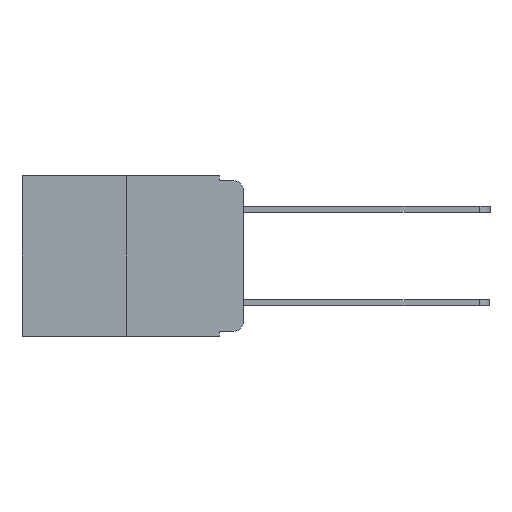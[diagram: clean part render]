
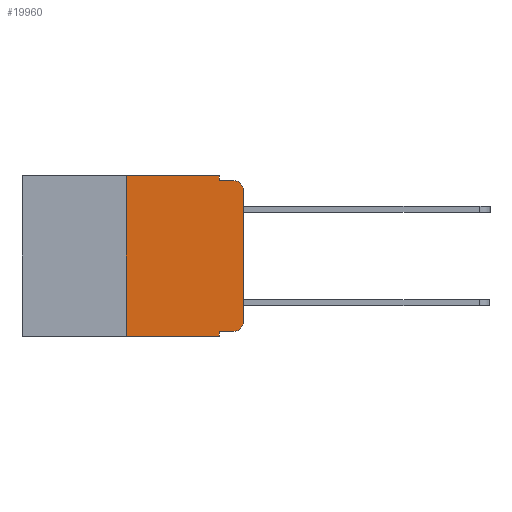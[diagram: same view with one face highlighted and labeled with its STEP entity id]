
A CAD part, left-side view. The second image highlights one B-rep face of the part: STEP entity #19960.
In plain terms, the highlighted planar face has unit normal (-1, 0, 0).
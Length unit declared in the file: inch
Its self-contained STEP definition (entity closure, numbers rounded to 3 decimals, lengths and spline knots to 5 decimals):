
#76 = LINE ( 'NONE', #2492, #4510 ) ;
#156 = ORIENTED_EDGE ( 'NONE', *, *, #2588, .F. ) ;
#288 = CARTESIAN_POINT ( 'NONE',  ( 0., 0.051, 0. ) ) ;
#314 = EDGE_CURVE ( 'NONE', #11053, #2908, #867, .T. ) ;
#435 = DIRECTION ( 'NONE',  ( 0., 0., -1. ) ) ;
#867 = CIRCLE ( 'NONE', #7590, 0.02 ) ;
#887 = CARTESIAN_POINT ( 'NONE',  ( 0., 0., 0. ) ) ;
#1005 = VERTEX_POINT ( 'NONE', #15264 ) ;
#1090 = CARTESIAN_POINT ( 'NONE',  ( 0., 0.051, -0.333 ) ) ;
#1467 = EDGE_CURVE ( 'NONE', #4015, #11053, #2107, .T. ) ;
#2075 = ORIENTED_EDGE ( 'NONE', *, *, #9707, .T. ) ;
#2107 = LINE ( 'NONE', #20034, #14259 ) ;
#2492 = CARTESIAN_POINT ( 'NONE',  ( 0., 0.051, -0.01 ) ) ;
#2574 = DIRECTION ( 'NONE',  ( 0., 0., 1. ) ) ;
#2588 = EDGE_CURVE ( 'NONE', #4015, #8609, #17088, .T. ) ;
#2833 = CARTESIAN_POINT ( 'NONE',  ( 0., 0.25, -0.343 ) ) ;
#2897 = CARTESIAN_POINT ( 'NONE',  ( 0., 0.051, 0. ) ) ;
#2908 = VERTEX_POINT ( 'NONE', #8271 ) ;
#2931 = FACE_OUTER_BOUND ( 'NONE', #17811, .T. ) ;
#3025 = VECTOR ( 'NONE', #12382, 39.37008 ) ;
#3194 = DIRECTION ( 'NONE',  ( 0., 0., -1. ) ) ;
#3526 = CARTESIAN_POINT ( 'NONE',  ( 0., 0.473, -0.343 ) ) ;
#3558 = EDGE_CURVE ( 'NONE', #14035, #4809, #14408, .T. ) ;
#3570 = ORIENTED_EDGE ( 'NONE', *, *, #3558, .F. ) ;
#3691 = EDGE_CURVE ( 'NONE', #13144, #14035, #5046, .T. ) ;
#4015 = VERTEX_POINT ( 'NONE', #1090 ) ;
#4058 = CARTESIAN_POINT ( 'NONE',  ( 0., 0.473, 0. ) ) ;
#4120 = DIRECTION ( 'NONE',  ( 0., -1., 0. ) ) ;
#4510 = VECTOR ( 'NONE', #4120, 39.37008 ) ;
#4751 = EDGE_CURVE ( 'NONE', #4809, #15263, #18718, .T. ) ;
#4809 = VERTEX_POINT ( 'NONE', #15557 ) ;
#5046 = LINE ( 'NONE', #6833, #20170 ) ;
#5075 = VECTOR ( 'NONE', #435, 39.37008 ) ;
#5101 = DIRECTION ( 'NONE',  ( 0., -1., 0. ) ) ;
#5231 = CARTESIAN_POINT ( 'NONE',  ( 0., 0.25, 0. ) ) ;
#5235 = CARTESIAN_POINT ( 'NONE',  ( 0., 0.051, -0.01 ) ) ;
#5453 = ORIENTED_EDGE ( 'NONE', *, *, #6877, .T. ) ;
#5658 = DIRECTION ( 'NONE',  ( 1., 0., 0. ) ) ;
#5820 = EDGE_CURVE ( 'NONE', #15263, #7409, #76, .T. ) ;
#5997 = VECTOR ( 'NONE', #2574, 39.37008 ) ;
#6628 = ORIENTED_EDGE ( 'NONE', *, *, #7955, .T. ) ;
#6833 = CARTESIAN_POINT ( 'NONE',  ( 0., 0.25, 0. ) ) ;
#6877 = EDGE_CURVE ( 'NONE', #1005, #7409, #9290, .T. ) ;
#7409 = VERTEX_POINT ( 'NONE', #16894 ) ;
#7526 = CARTESIAN_POINT ( 'NONE',  ( 0., 0.051, -0.343 ) ) ;
#7590 = AXIS2_PLACEMENT_3D ( 'NONE', #18315, #18486, #3194 ) ;
#7669 = DIRECTION ( 'NONE',  ( -1., 0., 0. ) ) ;
#7955 = EDGE_CURVE ( 'NONE', #2908, #1005, #13856, .T. ) ;
#7968 = ORIENTED_EDGE ( 'NONE', *, *, #5820, .F. ) ;
#8271 = CARTESIAN_POINT ( 'NONE',  ( 0., 0., -0.313 ) ) ;
#8452 = DIRECTION ( 'NONE',  ( 0., 0., 1. ) ) ;
#8609 = VERTEX_POINT ( 'NONE', #7526 ) ;
#9290 = CIRCLE ( 'NONE', #17833, 0.02 ) ;
#9707 = EDGE_CURVE ( 'NONE', #13144, #8609, #17148, .T. ) ;
#9716 = CARTESIAN_POINT ( 'NONE',  ( 0., 0.473, 0. ) ) ;
#10321 = ORIENTED_EDGE ( 'NONE', *, *, #1467, .T. ) ;
#11053 = VERTEX_POINT ( 'NONE', #17579 ) ;
#11264 = DIRECTION ( 'NONE',  ( 0., -1., 0. ) ) ;
#11588 = VECTOR ( 'NONE', #5101, 39.37008 ) ;
#11955 = ORIENTED_EDGE ( 'NONE', *, *, #3691, .F. ) ;
#12382 = DIRECTION ( 'NONE',  ( 0., 0., -1. ) ) ;
#13144 = VERTEX_POINT ( 'NONE', #2833 ) ;
#13496 = PLANE ( 'NONE',  #14965 ) ;
#13856 = LINE ( 'NONE', #887, #5997 ) ;
#13919 = VECTOR ( 'NONE', #11264, 39.37008 ) ;
#14035 = VERTEX_POINT ( 'NONE', #5231 ) ;
#14259 = VECTOR ( 'NONE', #16511, 39.37008 ) ;
#14408 = LINE ( 'NONE', #9716, #13919 ) ;
#14965 = AXIS2_PLACEMENT_3D ( 'NONE', #4058, #5658, #16613 ) ;
#15134 = ORIENTED_EDGE ( 'NONE', *, *, #4751, .F. ) ;
#15263 = VERTEX_POINT ( 'NONE', #5235 ) ;
#15264 = CARTESIAN_POINT ( 'NONE',  ( 0., 0., -0.03 ) ) ;
#15557 = CARTESIAN_POINT ( 'NONE',  ( 0., 0.051, 0. ) ) ;
#16511 = DIRECTION ( 'NONE',  ( 0., -1., 0. ) ) ;
#16613 = DIRECTION ( 'NONE',  ( 0., 0., -1. ) ) ;
#16894 = CARTESIAN_POINT ( 'NONE',  ( 0., 0.02, -0.01 ) ) ;
#16984 = CARTESIAN_POINT ( 'NONE',  ( 0., 0.02, -0.03 ) ) ;
#17088 = LINE ( 'NONE', #288, #5075 ) ;
#17148 = LINE ( 'NONE', #3526, #11588 ) ;
#17579 = CARTESIAN_POINT ( 'NONE',  ( 0., 0.02, -0.333 ) ) ;
#17811 = EDGE_LOOP ( 'NONE', ( #6628, #5453, #7968, #15134, #3570, #11955, #2075, #156, #10321, #18066 ) ) ;
#17833 = AXIS2_PLACEMENT_3D ( 'NONE', #16984, #7669, #18543 ) ;
#18066 = ORIENTED_EDGE ( 'NONE', *, *, #314, .T. ) ;
#18315 = CARTESIAN_POINT ( 'NONE',  ( 0., 0.02, -0.313 ) ) ;
#18486 = DIRECTION ( 'NONE',  ( -1., 0., 0. ) ) ;
#18543 = DIRECTION ( 'NONE',  ( 0., 0., -1. ) ) ;
#18718 = LINE ( 'NONE', #2897, #3025 ) ;
#19960 = ADVANCED_FACE ( 'NONE', ( #2931 ), #13496, .F. ) ;
#20034 = CARTESIAN_POINT ( 'NONE',  ( 0., 0.051, -0.333 ) ) ;
#20170 = VECTOR ( 'NONE', #8452, 39.37008 ) ;
